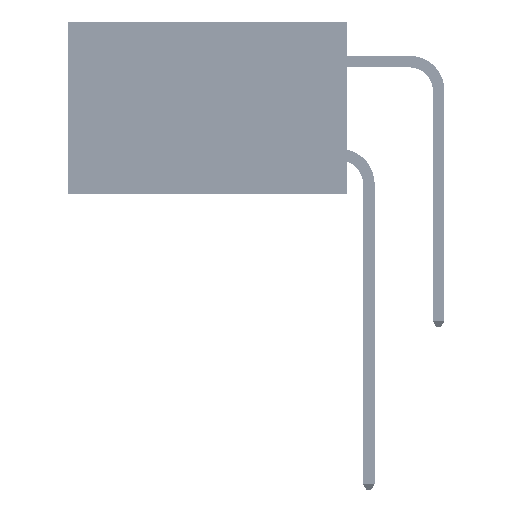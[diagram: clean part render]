
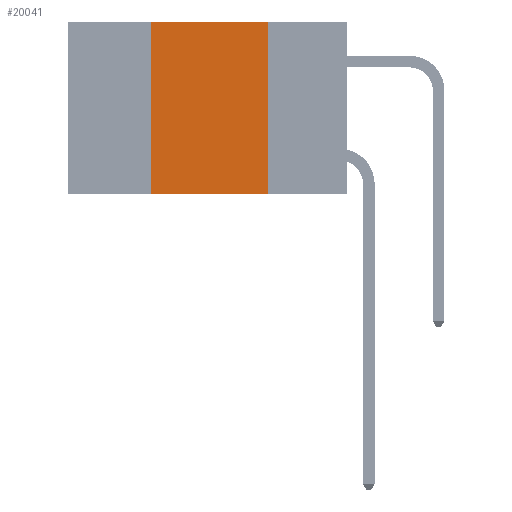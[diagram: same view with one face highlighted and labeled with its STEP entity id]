
A CAD part, left-side view. The second image highlights one B-rep face of the part: STEP entity #20041.
In plain terms, the highlighted planar face has unit normal (-1, 0, 0).
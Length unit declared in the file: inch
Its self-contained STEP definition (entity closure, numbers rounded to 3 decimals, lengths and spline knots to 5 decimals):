
#5818 = EDGE_CURVE ( 'NONE', #9128, #44674, #29031, .T. ) ;
#6203 = VERTEX_POINT ( 'NONE', #28376 ) ;
#7372 = CARTESIAN_POINT ( 'NONE',  ( 0., 0.6, 0. ) ) ;
#9128 = VERTEX_POINT ( 'NONE', #30494 ) ;
#9701 = CARTESIAN_POINT ( 'NONE',  ( 0., 0.17, 0. ) ) ;
#9827 = ORIENTED_EDGE ( 'NONE', *, *, #5818, .F. ) ;
#9926 = VECTOR ( 'NONE', #48286, 39.37008 ) ;
#14865 = VECTOR ( 'NONE', #31924, 39.37008 ) ;
#15661 = CARTESIAN_POINT ( 'NONE',  ( 0., 0.6, 0. ) ) ;
#15907 = DIRECTION ( 'NONE',  ( 1., 0., 0. ) ) ;
#18634 = LINE ( 'NONE', #25860, #35818 ) ;
#18712 = ORIENTED_EDGE ( 'NONE', *, *, #36687, .F. ) ;
#20041 = ADVANCED_FACE ( 'NONE', ( #27635 ), #43967, .F. ) ;
#20222 = CARTESIAN_POINT ( 'NONE',  ( 0., 0.42, 0. ) ) ;
#21369 = EDGE_CURVE ( 'NONE', #44674, #22081, #24447, .T. ) ;
#22081 = VERTEX_POINT ( 'NONE', #9701 ) ;
#22641 = DIRECTION ( 'NONE',  ( 0., 0., -1. ) ) ;
#24447 = LINE ( 'NONE', #15661, #14865 ) ;
#25860 = CARTESIAN_POINT ( 'NONE',  ( 0., 0.17, 0. ) ) ;
#27635 = FACE_OUTER_BOUND ( 'NONE', #46389, .T. ) ;
#28376 = CARTESIAN_POINT ( 'NONE',  ( 0., 0.17, -0.37 ) ) ;
#28402 = AXIS2_PLACEMENT_3D ( 'NONE', #7372, #15907, #36210 ) ;
#29031 = LINE ( 'NONE', #20222, #9926 ) ;
#30494 = CARTESIAN_POINT ( 'NONE',  ( 0., 0.42, -0.37 ) ) ;
#31924 = DIRECTION ( 'NONE',  ( 0., -1., 0. ) ) ;
#32499 = CARTESIAN_POINT ( 'NONE',  ( 0., 0.6, -0.37 ) ) ;
#32765 = LINE ( 'NONE', #32499, #34831 ) ;
#34831 = VECTOR ( 'NONE', #49071, 39.37008 ) ;
#35818 = VECTOR ( 'NONE', #22641, 39.37008 ) ;
#35913 = EDGE_CURVE ( 'NONE', #9128, #6203, #32765, .T. ) ;
#36210 = DIRECTION ( 'NONE',  ( 0., 0., -1. ) ) ;
#36687 = EDGE_CURVE ( 'NONE', #22081, #6203, #18634, .T. ) ;
#40690 = ORIENTED_EDGE ( 'NONE', *, *, #21369, .F. ) ;
#43900 = CARTESIAN_POINT ( 'NONE',  ( 0., 0.42, 0. ) ) ;
#43903 = ORIENTED_EDGE ( 'NONE', *, *, #35913, .T. ) ;
#43967 = PLANE ( 'NONE',  #28402 ) ;
#44674 = VERTEX_POINT ( 'NONE', #43900 ) ;
#46389 = EDGE_LOOP ( 'NONE', ( #18712, #40690, #9827, #43903 ) ) ;
#48286 = DIRECTION ( 'NONE',  ( 0., 0., 1. ) ) ;
#49071 = DIRECTION ( 'NONE',  ( 0., -1., 0. ) ) ;
